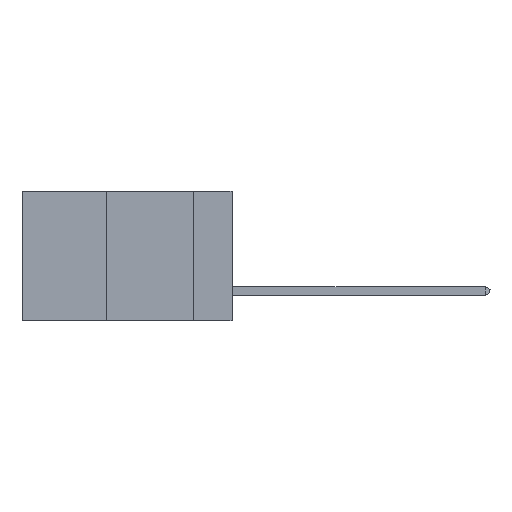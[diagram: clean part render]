
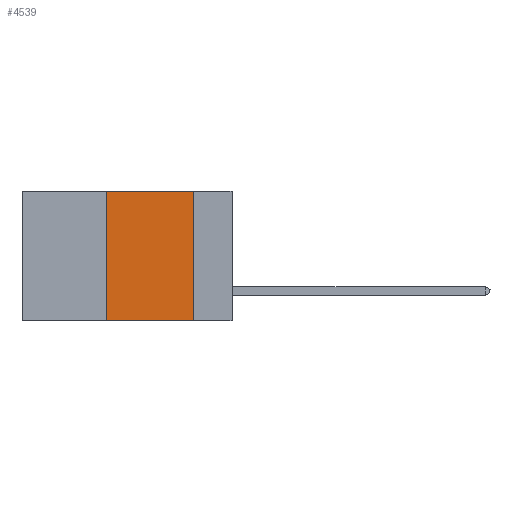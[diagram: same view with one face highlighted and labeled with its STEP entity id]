
A CAD part, left-side view. The second image highlights one B-rep face of the part: STEP entity #4539.
In plain terms, the highlighted planar face has unit normal (-1, 0, 0).
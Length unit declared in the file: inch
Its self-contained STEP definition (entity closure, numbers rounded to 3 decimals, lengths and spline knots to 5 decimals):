
#84 = CARTESIAN_POINT ( 'NONE',  ( 0., 0.6, 0. ) ) ;
#614 = EDGE_CURVE ( 'NONE', #9765, #5356, #3783, .T. ) ;
#630 = ORIENTED_EDGE ( 'NONE', *, *, #6698, .F. ) ;
#1258 = AXIS2_PLACEMENT_3D ( 'NONE', #84, #8666, #8538 ) ;
#1585 = CARTESIAN_POINT ( 'NONE',  ( 0., 0.36, 0. ) ) ;
#1788 = ORIENTED_EDGE ( 'NONE', *, *, #6676, .T. ) ;
#2179 = EDGE_LOOP ( 'NONE', ( #3666, #5334, #630, #1788 ) ) ;
#2399 = LINE ( 'NONE', #7026, #2893 ) ;
#2566 = DIRECTION ( 'NONE',  ( 0., 0., -1. ) ) ;
#2598 = VECTOR ( 'NONE', #2566, 39.37008 ) ;
#2893 = VECTOR ( 'NONE', #7300, 39.37008 ) ;
#3246 = CARTESIAN_POINT ( 'NONE',  ( 0., 0.6, 0. ) ) ;
#3666 = ORIENTED_EDGE ( 'NONE', *, *, #3679, .F. ) ;
#3679 = EDGE_CURVE ( 'NONE', #5356, #6846, #4274, .T. ) ;
#3783 = LINE ( 'NONE', #3246, #6897 ) ;
#4274 = LINE ( 'NONE', #5636, #2598 ) ;
#4539 = ADVANCED_FACE ( 'NONE', ( #6880 ), #4774, .F. ) ;
#4583 = CARTESIAN_POINT ( 'NONE',  ( 0., 0.36, -0.37 ) ) ;
#4774 = PLANE ( 'NONE',  #1258 ) ;
#5334 = ORIENTED_EDGE ( 'NONE', *, *, #614, .F. ) ;
#5356 = VERTEX_POINT ( 'NONE', #7959 ) ;
#5636 = CARTESIAN_POINT ( 'NONE',  ( 0., 0.11, 0. ) ) ;
#6582 = CARTESIAN_POINT ( 'NONE',  ( 0., 0.11, -0.37 ) ) ;
#6676 = EDGE_CURVE ( 'NONE', #9129, #6846, #8191, .T. ) ;
#6698 = EDGE_CURVE ( 'NONE', #9129, #9765, #2399, .T. ) ;
#6846 = VERTEX_POINT ( 'NONE', #6582 ) ;
#6880 = FACE_OUTER_BOUND ( 'NONE', #2179, .T. ) ;
#6897 = VECTOR ( 'NONE', #7046, 39.37008 ) ;
#7026 = CARTESIAN_POINT ( 'NONE',  ( 0., 0.36, 0. ) ) ;
#7046 = DIRECTION ( 'NONE',  ( 0., -1., 0. ) ) ;
#7300 = DIRECTION ( 'NONE',  ( 0., 0., 1. ) ) ;
#7878 = CARTESIAN_POINT ( 'NONE',  ( 0., 0.6, -0.37 ) ) ;
#7959 = CARTESIAN_POINT ( 'NONE',  ( 0., 0.11, 0. ) ) ;
#8191 = LINE ( 'NONE', #7878, #9492 ) ;
#8538 = DIRECTION ( 'NONE',  ( 0., 0., -1. ) ) ;
#8666 = DIRECTION ( 'NONE',  ( 1., 0., 0. ) ) ;
#8731 = DIRECTION ( 'NONE',  ( 0., -1., 0. ) ) ;
#9129 = VERTEX_POINT ( 'NONE', #4583 ) ;
#9492 = VECTOR ( 'NONE', #8731, 39.37008 ) ;
#9765 = VERTEX_POINT ( 'NONE', #1585 ) ;
